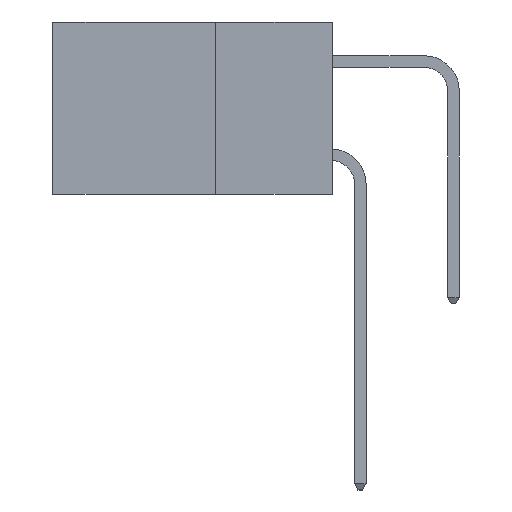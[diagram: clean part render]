
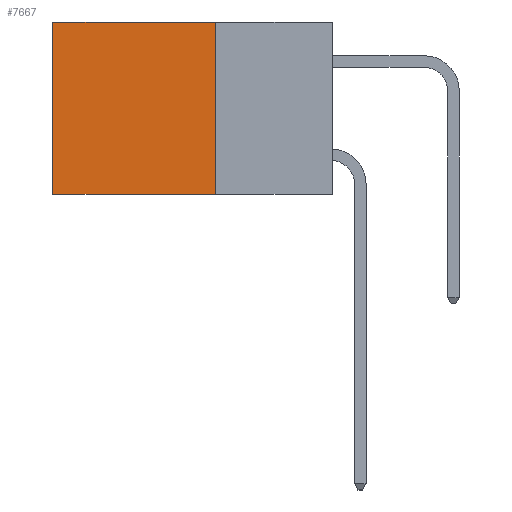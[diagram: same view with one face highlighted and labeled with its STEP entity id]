
A CAD part, left-side view. The second image highlights one B-rep face of the part: STEP entity #7667.
In plain terms, the highlighted planar face has unit normal (-1, 0, 0).
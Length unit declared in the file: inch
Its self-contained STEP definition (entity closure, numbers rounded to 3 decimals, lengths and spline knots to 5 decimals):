
#460 = VERTEX_POINT ( 'NONE', #10677 ) ;
#516 = EDGE_LOOP ( 'NONE', ( #7680, #10791, #9894, #11359 ) ) ;
#1690 = FACE_OUTER_BOUND ( 'NONE', #516, .T. ) ;
#2810 = VECTOR ( 'NONE', #5373, 39.37008 ) ;
#3216 = VERTEX_POINT ( 'NONE', #4441 ) ;
#4441 = CARTESIAN_POINT ( 'NONE',  ( 0.2615, 0.25, 0. ) ) ;
#4803 = VECTOR ( 'NONE', #5200, 39.37008 ) ;
#5200 = DIRECTION ( 'NONE',  ( 0., 0., -1. ) ) ;
#5213 = CARTESIAN_POINT ( 'NONE',  ( 0.2615, 0.6, -0.37 ) ) ;
#5373 = DIRECTION ( 'NONE',  ( 0., 0., -1. ) ) ;
#6531 = EDGE_CURVE ( 'NONE', #11115, #16910, #8518, .T. ) ;
#7350 = AXIS2_PLACEMENT_3D ( 'NONE', #9167, #8287, #8319 ) ;
#7667 = ADVANCED_FACE ( 'NONE', ( #1690 ), #7830, .F. ) ;
#7680 = ORIENTED_EDGE ( 'NONE', *, *, #6531, .T. ) ;
#7760 = CARTESIAN_POINT ( 'NONE',  ( 0.2615, 0.6, -0.37 ) ) ;
#7830 = PLANE ( 'NONE',  #7350 ) ;
#8107 = EDGE_CURVE ( 'NONE', #3216, #11115, #16207, .T. ) ;
#8142 = EDGE_CURVE ( 'NONE', #460, #16910, #12751, .T. ) ;
#8287 = DIRECTION ( 'NONE',  ( 1., 0., 0. ) ) ;
#8319 = DIRECTION ( 'NONE',  ( 0., 0., -1. ) ) ;
#8518 = LINE ( 'NONE', #5213, #4803 ) ;
#8839 = DIRECTION ( 'NONE',  ( 0., 1., 0. ) ) ;
#8863 = DIRECTION ( 'NONE',  ( 0., 1., 0. ) ) ;
#8877 = CARTESIAN_POINT ( 'NONE',  ( 0.2615, 0.25, 0. ) ) ;
#9064 = CARTESIAN_POINT ( 'NONE',  ( 0.2615, 0.25, -0.37 ) ) ;
#9167 = CARTESIAN_POINT ( 'NONE',  ( 0.2615, 0.25, -0.37 ) ) ;
#9894 = ORIENTED_EDGE ( 'NONE', *, *, #15972, .F. ) ;
#10677 = CARTESIAN_POINT ( 'NONE',  ( 0.2615, 0.25, -0.37 ) ) ;
#10791 = ORIENTED_EDGE ( 'NONE', *, *, #8142, .F. ) ;
#11115 = VERTEX_POINT ( 'NONE', #13665 ) ;
#11359 = ORIENTED_EDGE ( 'NONE', *, *, #8107, .T. ) ;
#12330 = VECTOR ( 'NONE', #8839, 39.37008 ) ;
#12751 = LINE ( 'NONE', #9064, #12330 ) ;
#13589 = VECTOR ( 'NONE', #8863, 39.37008 ) ;
#13665 = CARTESIAN_POINT ( 'NONE',  ( 0.2615, 0.6, 0. ) ) ;
#14948 = CARTESIAN_POINT ( 'NONE',  ( 0.2615, 0.25, -0.37 ) ) ;
#15972 = EDGE_CURVE ( 'NONE', #3216, #460, #16813, .T. ) ;
#16207 = LINE ( 'NONE', #8877, #13589 ) ;
#16813 = LINE ( 'NONE', #14948, #2810 ) ;
#16910 = VERTEX_POINT ( 'NONE', #7760 ) ;
